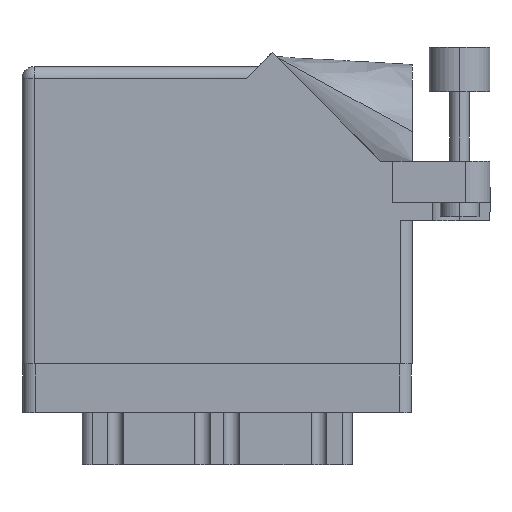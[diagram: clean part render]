
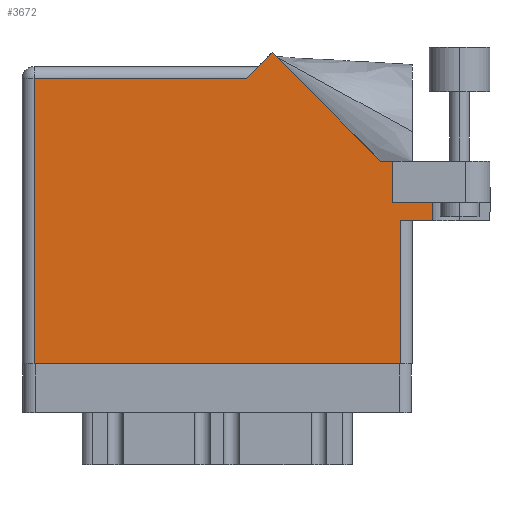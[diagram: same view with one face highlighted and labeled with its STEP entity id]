
A CAD part, front view. The second image highlights one B-rep face of the part: STEP entity #3672.
In plain terms, the highlighted face is planar.
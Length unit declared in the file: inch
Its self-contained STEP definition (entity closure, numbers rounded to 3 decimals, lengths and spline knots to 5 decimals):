
#172 = CARTESIAN_POINT ( 'NONE',  ( 0., 0., 0. ) ) ;
#345 = LINE ( 'NONE', #27012, #21100 ) ;
#527 = LINE ( 'NONE', #25003, #23129 ) ;
#1701 = DIRECTION ( 'NONE',  ( -0.707, -0.707, 0. ) ) ;
#2319 = CARTESIAN_POINT ( 'NONE',  ( 2.1115, 0.831, 0. ) ) ;
#3606 = EDGE_CURVE ( 'NONE', #19316, #33167, #20232, .T. ) ;
#3672 = ADVANCED_FACE ( 'NONE', ( #18231 ), #39020, .F. ) ;
#3749 = VERTEX_POINT ( 'NONE', #27138 ) ;
#5184 = LINE ( 'NONE', #11129, #31242 ) ;
#5782 = DIRECTION ( 'NONE',  ( 1., 0., 0. ) ) ;
#6193 = LINE ( 'NONE', #36051, #26539 ) ;
#6485 = CARTESIAN_POINT ( 'NONE',  ( 1.155, 1.468, 0. ) ) ;
#6520 = ORIENTED_EDGE ( 'NONE', *, *, #3606, .T. ) ;
#7095 = EDGE_LOOP ( 'NONE', ( #28911, #28905, #19250, #17436, #29432, #15804, #35174, #18520, #6520, #35682, #12977 ) ) ;
#7449 = VERTEX_POINT ( 'NONE', #9224 ) ;
#7731 = CARTESIAN_POINT ( 'NONE',  ( 1.91, 0.831, 0. ) ) ;
#7752 = DIRECTION ( 'NONE',  ( 0., -1., 0. ) ) ;
#7875 = VECTOR ( 'NONE', #1701, 39.37008 ) ;
#9222 = CARTESIAN_POINT ( 'NONE',  ( 2.1115, 1.16177, 0. ) ) ;
#9224 = CARTESIAN_POINT ( 'NONE',  ( 1.84442, 1.044, 0. ) ) ;
#9256 = CARTESIAN_POINT ( 'NONE',  ( 1.28771, 1.60071, 0. ) ) ;
#11129 = CARTESIAN_POINT ( 'NONE',  ( 2.01, 0.737, 0. ) ) ;
#11552 = DIRECTION ( 'NONE',  ( -1., 0., 0. ) ) ;
#11603 = EDGE_CURVE ( 'NONE', #16463, #17711, #26803, .T. ) ;
#11850 = LINE ( 'NONE', #172, #30481 ) ;
#12337 = CARTESIAN_POINT ( 'NONE',  ( 2.1115, 0.737, 0. ) ) ;
#12581 = CARTESIAN_POINT ( 'NONE',  ( 1.948, 0.737, 0. ) ) ;
#12796 = EDGE_CURVE ( 'NONE', #22834, #20627, #20100, .T. ) ;
#12939 = AXIS2_PLACEMENT_3D ( 'NONE', #33085, #17661, #11552 ) ;
#12977 = ORIENTED_EDGE ( 'NONE', *, *, #13699, .T. ) ;
#12992 = EDGE_CURVE ( 'NONE', #7449, #19316, #345, .T. ) ;
#13695 = DIRECTION ( 'NONE',  ( 1., 0., 0. ) ) ;
#13699 = EDGE_CURVE ( 'NONE', #3749, #25601, #36646, .T. ) ;
#15804 = ORIENTED_EDGE ( 'NONE', *, *, #12796, .T. ) ;
#16463 = VERTEX_POINT ( 'NONE', #2319 ) ;
#17436 = ORIENTED_EDGE ( 'NONE', *, *, #11603, .F. ) ;
#17661 = DIRECTION ( 'NONE',  ( 0., 0., -1. ) ) ;
#17711 = VERTEX_POINT ( 'NONE', #12337 ) ;
#18231 = FACE_OUTER_BOUND ( 'NONE', #7095, .T. ) ;
#18520 = ORIENTED_EDGE ( 'NONE', *, *, #12992, .T. ) ;
#19250 = ORIENTED_EDGE ( 'NONE', *, *, #25159, .T. ) ;
#19316 = VERTEX_POINT ( 'NONE', #9256 ) ;
#19712 = VECTOR ( 'NONE', #7752, 39.37008 ) ;
#20100 = LINE ( 'NONE', #37916, #22985 ) ;
#20196 = EDGE_CURVE ( 'NONE', #33167, #3749, #6193, .T. ) ;
#20232 = LINE ( 'NONE', #32312, #7875 ) ;
#20457 = VECTOR ( 'NONE', #30178, 39.37008 ) ;
#20548 = LINE ( 'NONE', #35794, #25662 ) ;
#20627 = VERTEX_POINT ( 'NONE', #27224 ) ;
#21100 = VECTOR ( 'NONE', #24626, 39.37008 ) ;
#21609 = CARTESIAN_POINT ( 'NONE',  ( 0.062, 0., 0. ) ) ;
#21635 = LINE ( 'NONE', #7731, #34940 ) ;
#22834 = VERTEX_POINT ( 'NONE', #24659 ) ;
#22985 = VECTOR ( 'NONE', #23073, 39.37008 ) ;
#23073 = DIRECTION ( 'NONE',  ( 0., 1., 0. ) ) ;
#23129 = VECTOR ( 'NONE', #34109, 39.37008 ) ;
#23132 = CARTESIAN_POINT ( 'NONE',  ( 0.062, 0., 0. ) ) ;
#23244 = VERTEX_POINT ( 'NONE', #12581 ) ;
#23872 = EDGE_CURVE ( 'NONE', #27243, #23244, #20548, .T. ) ;
#24085 = DIRECTION ( 'NONE',  ( 0., 1., 0. ) ) ;
#24626 = DIRECTION ( 'NONE',  ( -0.707, 0.707, 0. ) ) ;
#24659 = CARTESIAN_POINT ( 'NONE',  ( 1.91, 0.831, 0. ) ) ;
#25003 = CARTESIAN_POINT ( 'NONE',  ( 2.41, 1.044, 0. ) ) ;
#25159 = EDGE_CURVE ( 'NONE', #23244, #17711, #5184, .T. ) ;
#25601 = VERTEX_POINT ( 'NONE', #23132 ) ;
#25662 = VECTOR ( 'NONE', #24085, 39.37008 ) ;
#26539 = VECTOR ( 'NONE', #29719, 39.37008 ) ;
#26803 = LINE ( 'NONE', #9222, #20457 ) ;
#26844 = DIRECTION ( 'NONE',  ( 1., 0., 0. ) ) ;
#27012 = CARTESIAN_POINT ( 'NONE',  ( 1.84442, 1.044, 0. ) ) ;
#27138 = CARTESIAN_POINT ( 'NONE',  ( 0.062, 1.468, 0. ) ) ;
#27224 = CARTESIAN_POINT ( 'NONE',  ( 1.91, 1.044, 0. ) ) ;
#27243 = VERTEX_POINT ( 'NONE', #35724 ) ;
#27424 = EDGE_CURVE ( 'NONE', #20627, #7449, #527, .T. ) ;
#28905 = ORIENTED_EDGE ( 'NONE', *, *, #23872, .T. ) ;
#28911 = ORIENTED_EDGE ( 'NONE', *, *, #37206, .T. ) ;
#29432 = ORIENTED_EDGE ( 'NONE', *, *, #37843, .F. ) ;
#29719 = DIRECTION ( 'NONE',  ( -1., 0., 0. ) ) ;
#30178 = DIRECTION ( 'NONE',  ( 0., -1., 0. ) ) ;
#30481 = VECTOR ( 'NONE', #26844, 39.37008 ) ;
#31242 = VECTOR ( 'NONE', #5782, 39.37008 ) ;
#32312 = CARTESIAN_POINT ( 'NONE',  ( 1.217, 1.53, 0. ) ) ;
#33085 = CARTESIAN_POINT ( 'NONE',  ( 0., 1.53, 0. ) ) ;
#33167 = VERTEX_POINT ( 'NONE', #6485 ) ;
#34109 = DIRECTION ( 'NONE',  ( -1., 0., 0. ) ) ;
#34940 = VECTOR ( 'NONE', #13695, 39.37008 ) ;
#35174 = ORIENTED_EDGE ( 'NONE', *, *, #27424, .T. ) ;
#35682 = ORIENTED_EDGE ( 'NONE', *, *, #20196, .T. ) ;
#35724 = CARTESIAN_POINT ( 'NONE',  ( 1.948, 0., 0. ) ) ;
#35794 = CARTESIAN_POINT ( 'NONE',  ( 1.948, 0.737, 0. ) ) ;
#36051 = CARTESIAN_POINT ( 'NONE',  ( 0., 1.468, 0. ) ) ;
#36646 = LINE ( 'NONE', #21609, #19712 ) ;
#37206 = EDGE_CURVE ( 'NONE', #25601, #27243, #11850, .T. ) ;
#37843 = EDGE_CURVE ( 'NONE', #22834, #16463, #21635, .T. ) ;
#37916 = CARTESIAN_POINT ( 'NONE',  ( 1.91, 0.831, 0. ) ) ;
#39020 = PLANE ( 'NONE',  #12939 ) ;
